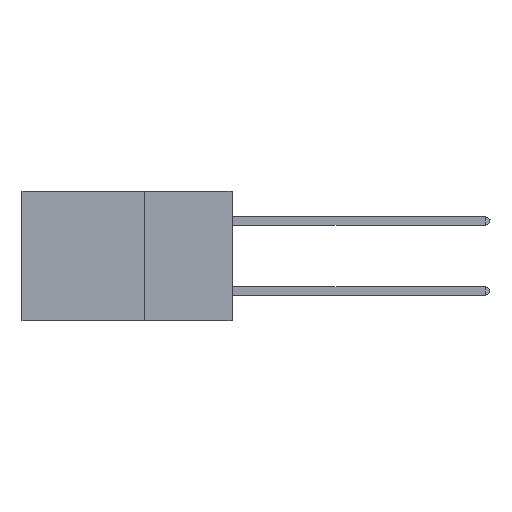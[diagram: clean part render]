
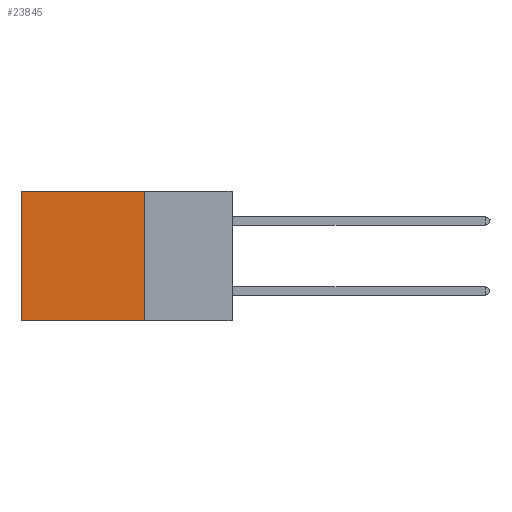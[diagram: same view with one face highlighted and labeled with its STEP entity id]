
A CAD part, left-side view. The second image highlights one B-rep face of the part: STEP entity #23845.
In plain terms, the highlighted planar face has unit normal (-1, 0, 0).
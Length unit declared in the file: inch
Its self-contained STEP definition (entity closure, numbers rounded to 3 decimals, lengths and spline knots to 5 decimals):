
#1067 = VECTOR ( 'NONE', #24795, 39.37008 ) ;
#2242 = ORIENTED_EDGE ( 'NONE', *, *, #25841, .F. ) ;
#3115 = CARTESIAN_POINT ( 'NONE',  ( 0.2875, 0.25, 0. ) ) ;
#5671 = CARTESIAN_POINT ( 'NONE',  ( 0.2875, 0.6, -0.37 ) ) ;
#5688 = VECTOR ( 'NONE', #25087, 39.37008 ) ;
#5731 = VERTEX_POINT ( 'NONE', #3115 ) ;
#5976 = VERTEX_POINT ( 'NONE', #5671 ) ;
#8406 = EDGE_LOOP ( 'NONE', ( #36514, #2242, #21781, #19299 ) ) ;
#9568 = EDGE_CURVE ( 'NONE', #5731, #25817, #26123, .T. ) ;
#10517 = CARTESIAN_POINT ( 'NONE',  ( 0.2875, 0.25, -0.37 ) ) ;
#11277 = CARTESIAN_POINT ( 'NONE',  ( 0.2875, 0.25, 0. ) ) ;
#12260 = CARTESIAN_POINT ( 'NONE',  ( 0.2875, 0.25, 0. ) ) ;
#14454 = AXIS2_PLACEMENT_3D ( 'NONE', #12260, #19979, #23489 ) ;
#16917 = FACE_OUTER_BOUND ( 'NONE', #8406, .T. ) ;
#17325 = CARTESIAN_POINT ( 'NONE',  ( 0.2875, 0.25, -0.37 ) ) ;
#19299 = ORIENTED_EDGE ( 'NONE', *, *, #27733, .T. ) ;
#19979 = DIRECTION ( 'NONE',  ( 1., 0., 0. ) ) ;
#21781 = ORIENTED_EDGE ( 'NONE', *, *, #9568, .F. ) ;
#23489 = DIRECTION ( 'NONE',  ( 0., 0., -1. ) ) ;
#23845 = ADVANCED_FACE ( 'NONE', ( #16917 ), #41494, .F. ) ;
#24795 = DIRECTION ( 'NONE',  ( 0., 1., 0. ) ) ;
#25087 = DIRECTION ( 'NONE',  ( 0., 1., 0. ) ) ;
#25817 = VERTEX_POINT ( 'NONE', #17325 ) ;
#25841 = EDGE_CURVE ( 'NONE', #25817, #5976, #42123, .T. ) ;
#26123 = LINE ( 'NONE', #30082, #37154 ) ;
#27733 = EDGE_CURVE ( 'NONE', #5731, #39258, #35387, .T. ) ;
#28503 = CARTESIAN_POINT ( 'NONE',  ( 0.2875, 0.6, 0. ) ) ;
#29404 = DIRECTION ( 'NONE',  ( 0., 0., -1. ) ) ;
#30082 = CARTESIAN_POINT ( 'NONE',  ( 0.2875, 0.25, 0. ) ) ;
#34542 = VECTOR ( 'NONE', #42769, 39.37008 ) ;
#35387 = LINE ( 'NONE', #11277, #5688 ) ;
#36424 = CARTESIAN_POINT ( 'NONE',  ( 0.2875, 0.6, 0. ) ) ;
#36514 = ORIENTED_EDGE ( 'NONE', *, *, #44767, .T. ) ;
#37154 = VECTOR ( 'NONE', #29404, 39.37008 ) ;
#39258 = VERTEX_POINT ( 'NONE', #36424 ) ;
#41494 = PLANE ( 'NONE',  #14454 ) ;
#42123 = LINE ( 'NONE', #10517, #1067 ) ;
#42769 = DIRECTION ( 'NONE',  ( 0., 0., -1. ) ) ;
#44767 = EDGE_CURVE ( 'NONE', #39258, #5976, #45819, .T. ) ;
#45819 = LINE ( 'NONE', #28503, #34542 ) ;
